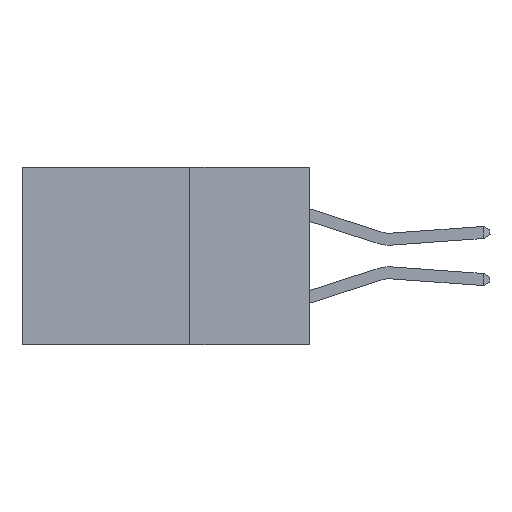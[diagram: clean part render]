
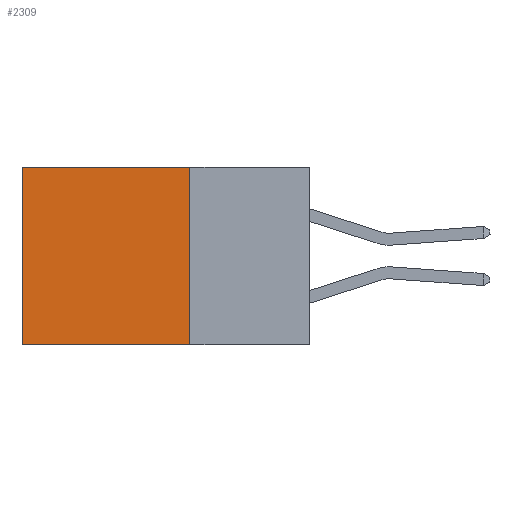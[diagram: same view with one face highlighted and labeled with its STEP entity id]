
A CAD part, left-side view. The second image highlights one B-rep face of the part: STEP entity #2309.
In plain terms, the highlighted planar face has unit normal (-1, 0, 0).
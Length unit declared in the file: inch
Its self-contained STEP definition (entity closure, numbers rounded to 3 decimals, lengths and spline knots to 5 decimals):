
#73 = CARTESIAN_POINT ( 'NONE',  ( 0.298, 0.25, 0. ) ) ;
#145 = CARTESIAN_POINT ( 'NONE',  ( 0.298, 0.25, 0. ) ) ;
#220 = PLANE ( 'NONE',  #4779 ) ;
#254 = EDGE_CURVE ( 'NONE', #3965, #609, #7866, .T. ) ;
#609 = VERTEX_POINT ( 'NONE', #11092 ) ;
#1134 = CARTESIAN_POINT ( 'NONE',  ( 0.298, 0.25, 0. ) ) ;
#1229 = DIRECTION ( 'NONE',  ( 0., 1., 0. ) ) ;
#1913 = DIRECTION ( 'NONE',  ( 0., 0., -1. ) ) ;
#1927 = DIRECTION ( 'NONE',  ( 0., 1., 0. ) ) ;
#1961 = EDGE_CURVE ( 'NONE', #8343, #609, #9682, .T. ) ;
#2181 = ORIENTED_EDGE ( 'NONE', *, *, #11738, .T. ) ;
#2309 = ADVANCED_FACE ( 'NONE', ( #5921 ), #220, .F. ) ;
#2770 = ORIENTED_EDGE ( 'NONE', *, *, #8214, .F. ) ;
#2883 = LINE ( 'NONE', #73, #7492 ) ;
#3064 = VECTOR ( 'NONE', #1229, 39.37008 ) ;
#3304 = ORIENTED_EDGE ( 'NONE', *, *, #1961, .F. ) ;
#3719 = CARTESIAN_POINT ( 'NONE',  ( 0.298, 0.6, 0. ) ) ;
#3962 = VERTEX_POINT ( 'NONE', #145 ) ;
#3965 = VERTEX_POINT ( 'NONE', #3719 ) ;
#4531 = DIRECTION ( 'NONE',  ( 0., 0., -1. ) ) ;
#4779 = AXIS2_PLACEMENT_3D ( 'NONE', #1134, #7550, #11245 ) ;
#5496 = CARTESIAN_POINT ( 'NONE',  ( 0.298, 0.25, 0. ) ) ;
#5808 = LINE ( 'NONE', #5496, #10579 ) ;
#5921 = FACE_OUTER_BOUND ( 'NONE', #6987, .T. ) ;
#6616 = CARTESIAN_POINT ( 'NONE',  ( 0.298, 0.25, -0.37 ) ) ;
#6671 = CARTESIAN_POINT ( 'NONE',  ( 0.298, 0.25, -0.37 ) ) ;
#6987 = EDGE_LOOP ( 'NONE', ( #11203, #3304, #2770, #2181 ) ) ;
#7492 = VECTOR ( 'NONE', #4531, 39.37008 ) ;
#7550 = DIRECTION ( 'NONE',  ( 1., 0., 0. ) ) ;
#7866 = LINE ( 'NONE', #10997, #11753 ) ;
#8214 = EDGE_CURVE ( 'NONE', #3962, #8343, #2883, .T. ) ;
#8343 = VERTEX_POINT ( 'NONE', #6671 ) ;
#9682 = LINE ( 'NONE', #6616, #3064 ) ;
#10579 = VECTOR ( 'NONE', #1927, 39.37008 ) ;
#10997 = CARTESIAN_POINT ( 'NONE',  ( 0.298, 0.6, 0. ) ) ;
#11092 = CARTESIAN_POINT ( 'NONE',  ( 0.298, 0.6, -0.37 ) ) ;
#11203 = ORIENTED_EDGE ( 'NONE', *, *, #254, .T. ) ;
#11245 = DIRECTION ( 'NONE',  ( 0., 0., -1. ) ) ;
#11738 = EDGE_CURVE ( 'NONE', #3962, #3965, #5808, .T. ) ;
#11753 = VECTOR ( 'NONE', #1913, 39.37008 ) ;
